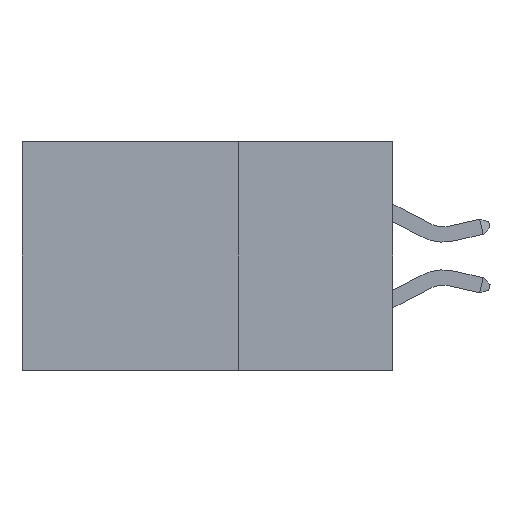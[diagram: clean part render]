
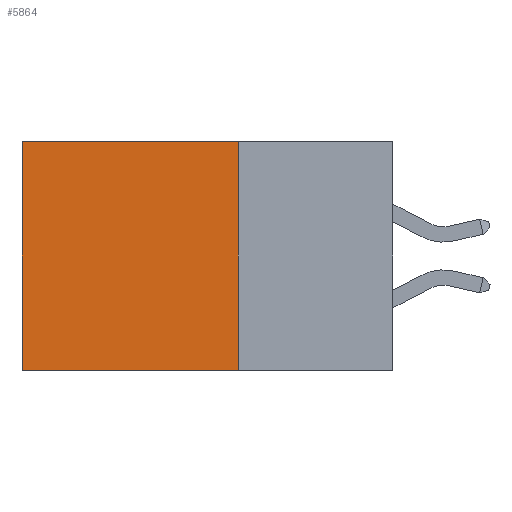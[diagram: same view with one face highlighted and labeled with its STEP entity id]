
A CAD part, left-side view. The second image highlights one B-rep face of the part: STEP entity #5864.
In plain terms, the highlighted planar face has unit normal (-1, 0, 0).
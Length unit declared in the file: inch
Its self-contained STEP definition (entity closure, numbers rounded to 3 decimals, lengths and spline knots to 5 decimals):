
#1427 = CARTESIAN_POINT ( 'NONE',  ( 0.2875, 0.25, 0. ) ) ;
#2594 = DIRECTION ( 'NONE',  ( 0., 0., -1. ) ) ;
#2666 = ORIENTED_EDGE ( 'NONE', *, *, #5429, .F. ) ;
#3252 = VECTOR ( 'NONE', #16876, 39.37008 ) ;
#3451 = PLANE ( 'NONE',  #3614 ) ;
#3614 = AXIS2_PLACEMENT_3D ( 'NONE', #13566, #15004, #6427 ) ;
#3984 = CARTESIAN_POINT ( 'NONE',  ( 0.2875, 0.6, -0.37 ) ) ;
#5429 = EDGE_CURVE ( 'NONE', #9971, #10854, #17204, .T. ) ;
#5864 = ADVANCED_FACE ( 'NONE', ( #17185 ), #3451, .F. ) ;
#6427 = DIRECTION ( 'NONE',  ( 0., 0., -1. ) ) ;
#6506 = EDGE_CURVE ( 'NONE', #9971, #10682, #18273, .T. ) ;
#6526 = DIRECTION ( 'NONE',  ( 0., 1., 0. ) ) ;
#6863 = CARTESIAN_POINT ( 'NONE',  ( 0.2875, 0.25, 0. ) ) ;
#7458 = CARTESIAN_POINT ( 'NONE',  ( 0.2875, 0.25, 0. ) ) ;
#9971 = VERTEX_POINT ( 'NONE', #7458 ) ;
#10183 = DIRECTION ( 'NONE',  ( 0., 1., 0. ) ) ;
#10414 = LINE ( 'NONE', #11237, #14680 ) ;
#10682 = VERTEX_POINT ( 'NONE', #14780 ) ;
#10854 = VERTEX_POINT ( 'NONE', #12283 ) ;
#11237 = CARTESIAN_POINT ( 'NONE',  ( 0.2875, 0.6, 0. ) ) ;
#11361 = ORIENTED_EDGE ( 'NONE', *, *, #12076, .F. ) ;
#11831 = ORIENTED_EDGE ( 'NONE', *, *, #18074, .T. ) ;
#12076 = EDGE_CURVE ( 'NONE', #10854, #14991, #12385, .T. ) ;
#12186 = EDGE_LOOP ( 'NONE', ( #11831, #11361, #2666, #14816 ) ) ;
#12283 = CARTESIAN_POINT ( 'NONE',  ( 0.2875, 0.25, -0.37 ) ) ;
#12385 = LINE ( 'NONE', #17959, #15736 ) ;
#13566 = CARTESIAN_POINT ( 'NONE',  ( 0.2875, 0.25, 0. ) ) ;
#14517 = VECTOR ( 'NONE', #10183, 39.37008 ) ;
#14680 = VECTOR ( 'NONE', #2594, 39.37008 ) ;
#14780 = CARTESIAN_POINT ( 'NONE',  ( 0.2875, 0.6, 0. ) ) ;
#14816 = ORIENTED_EDGE ( 'NONE', *, *, #6506, .T. ) ;
#14991 = VERTEX_POINT ( 'NONE', #3984 ) ;
#15004 = DIRECTION ( 'NONE',  ( 1., 0., 0. ) ) ;
#15736 = VECTOR ( 'NONE', #6526, 39.37008 ) ;
#16876 = DIRECTION ( 'NONE',  ( 0., 0., -1. ) ) ;
#17185 = FACE_OUTER_BOUND ( 'NONE', #12186, .T. ) ;
#17204 = LINE ( 'NONE', #6863, #3252 ) ;
#17959 = CARTESIAN_POINT ( 'NONE',  ( 0.2875, 0.25, -0.37 ) ) ;
#18074 = EDGE_CURVE ( 'NONE', #10682, #14991, #10414, .T. ) ;
#18273 = LINE ( 'NONE', #1427, #14517 ) ;
